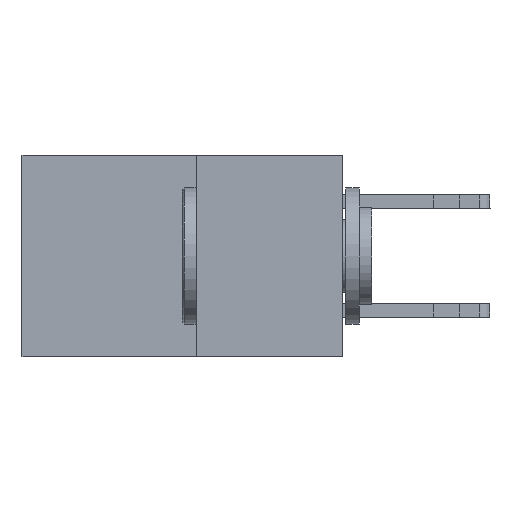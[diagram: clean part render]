
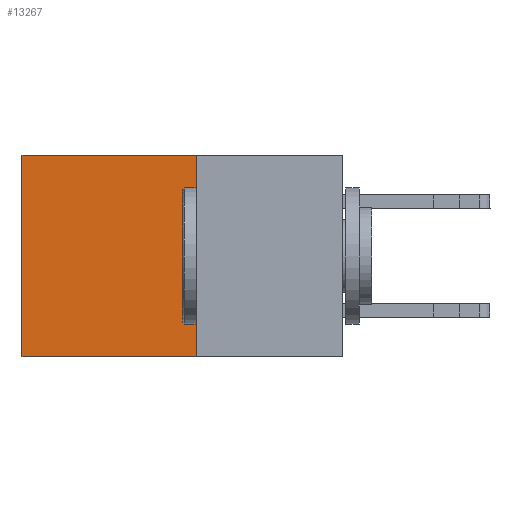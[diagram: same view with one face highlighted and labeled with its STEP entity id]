
A CAD part, left-side view. The second image highlights one B-rep face of the part: STEP entity #13267.
In plain terms, the highlighted planar face has unit normal (-1, 0, 0).
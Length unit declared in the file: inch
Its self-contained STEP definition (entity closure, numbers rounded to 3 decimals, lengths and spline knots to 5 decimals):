
#907 = AXIS2_PLACEMENT_3D ( 'NONE', #8876, #6043, #15862 ) ;
#1884 = CARTESIAN_POINT ( 'NONE',  ( 0.277, 0.27, -0.37 ) ) ;
#1916 = LINE ( 'NONE', #15008, #8657 ) ;
#2713 = LINE ( 'NONE', #5558, #17206 ) ;
#3331 = DIRECTION ( 'NONE',  ( 0., 1., 0. ) ) ;
#4138 = CARTESIAN_POINT ( 'NONE',  ( 0.277, 0.27, -0.37 ) ) ;
#4299 = VECTOR ( 'NONE', #5565, 39.37008 ) ;
#5462 = DIRECTION ( 'NONE',  ( 0., 0., -1. ) ) ;
#5558 = CARTESIAN_POINT ( 'NONE',  ( 0.277, 0.59, -0.37 ) ) ;
#5565 = DIRECTION ( 'NONE',  ( 0., 0., -1. ) ) ;
#5779 = ORIENTED_EDGE ( 'NONE', *, *, #14214, .F. ) ;
#5955 = ORIENTED_EDGE ( 'NONE', *, *, #6048, .T. ) ;
#6043 = DIRECTION ( 'NONE',  ( 1., 0., 0. ) ) ;
#6048 = EDGE_CURVE ( 'NONE', #12940, #17458, #2713, .T. ) ;
#7189 = CARTESIAN_POINT ( 'NONE',  ( 0.277, 0.27, -0.37 ) ) ;
#7915 = DIRECTION ( 'NONE',  ( 0., 1., 0. ) ) ;
#8083 = ORIENTED_EDGE ( 'NONE', *, *, #16110, .F. ) ;
#8657 = VECTOR ( 'NONE', #7915, 39.37008 ) ;
#8876 = CARTESIAN_POINT ( 'NONE',  ( 0.277, 0.27, -0.37 ) ) ;
#9011 = LINE ( 'NONE', #4138, #4299 ) ;
#9627 = ORIENTED_EDGE ( 'NONE', *, *, #16267, .T. ) ;
#10270 = CARTESIAN_POINT ( 'NONE',  ( 0.277, 0.59, -0.37 ) ) ;
#10429 = VERTEX_POINT ( 'NONE', #17701 ) ;
#11296 = VECTOR ( 'NONE', #3331, 39.37008 ) ;
#11352 = EDGE_LOOP ( 'NONE', ( #5955, #8083, #5779, #9627 ) ) ;
#12473 = CARTESIAN_POINT ( 'NONE',  ( 0.277, 0.59, 0. ) ) ;
#12940 = VERTEX_POINT ( 'NONE', #12473 ) ;
#13044 = FACE_OUTER_BOUND ( 'NONE', #11352, .T. ) ;
#13267 = ADVANCED_FACE ( 'NONE', ( #13044 ), #14582, .F. ) ;
#14214 = EDGE_CURVE ( 'NONE', #10429, #15394, #9011, .T. ) ;
#14582 = PLANE ( 'NONE',  #907 ) ;
#15008 = CARTESIAN_POINT ( 'NONE',  ( 0.277, 0.27, 0. ) ) ;
#15049 = LINE ( 'NONE', #1884, #11296 ) ;
#15394 = VERTEX_POINT ( 'NONE', #7189 ) ;
#15862 = DIRECTION ( 'NONE',  ( 0., 0., -1. ) ) ;
#16110 = EDGE_CURVE ( 'NONE', #15394, #17458, #15049, .T. ) ;
#16267 = EDGE_CURVE ( 'NONE', #10429, #12940, #1916, .T. ) ;
#17206 = VECTOR ( 'NONE', #5462, 39.37008 ) ;
#17458 = VERTEX_POINT ( 'NONE', #10270 ) ;
#17701 = CARTESIAN_POINT ( 'NONE',  ( 0.277, 0.27, 0. ) ) ;
